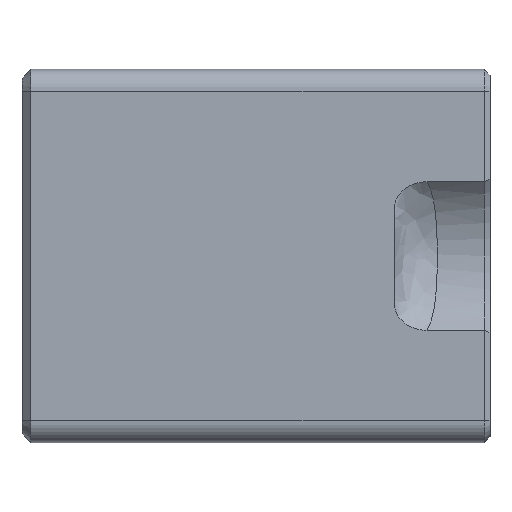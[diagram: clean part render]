
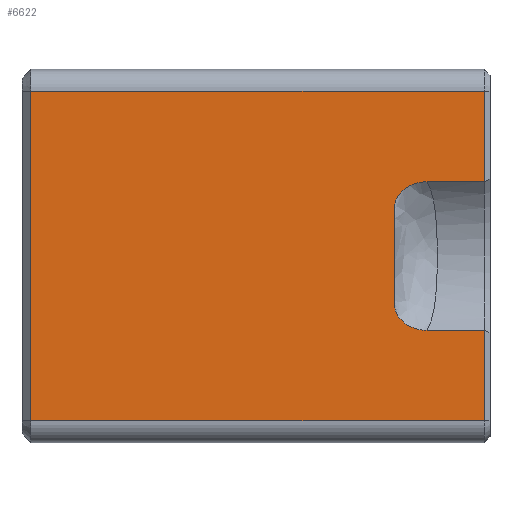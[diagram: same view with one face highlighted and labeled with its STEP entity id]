
A CAD part, front view. The second image highlights one B-rep face of the part: STEP entity #6622.
In plain terms, the highlighted planar face has unit normal (0, -1, 0).
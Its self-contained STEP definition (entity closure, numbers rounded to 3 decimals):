
#602=B_SPLINE_CURVE_WITH_KNOTS('',3,(#15782,#15783,#15784,#15785,#15786,
#15787,#15788,#15789,#15790,#15791,#15792,#15793,#15794,#15795,#15796,#15797,
#15798,#15799,#15800,#15801),.UNSPECIFIED.,.F.,.F.,(4,2,2,2,2,2,2,2,2,4),
(0.,0.,0.,0.002,0.007,
0.018,0.04,0.085,0.157,
0.234),.UNSPECIFIED.);
#603=B_SPLINE_CURVE_WITH_KNOTS('',3,(#15805,#15806,#15807,#15808,#15809,
#15810,#15811,#15812,#15813,#15814,#15815,#15816,#15817,#15818,#15819,#15820,
#15821,#15822,#15823,#15824),.UNSPECIFIED.,.F.,.F.,(4,2,2,2,2,2,2,2,2,4),
(0.,0.102,0.197,0.257,0.286,
0.3,0.306,0.31,0.31,
0.31),.UNSPECIFIED.);
#751=PLANE('',#7145);
#1197=FACE_OUTER_BOUND('',#1611,.T.);
#1611=EDGE_LOOP('',(#5960,#5961,#5962,#5963,#5964,#5965,#5966,#5967,#5968,
#5969));
#1972=LINE('',#15749,#2325);
#1981=LINE('',#15771,#2334);
#1982=LINE('',#15776,#2335);
#1983=LINE('',#15780,#2336);
#1984=LINE('',#15803,#2337);
#1985=LINE('',#15825,#2338);
#1986=LINE('',#15827,#2339);
#1987=LINE('',#15828,#2340);
#2325=VECTOR('',#8347,10.);
#2334=VECTOR('',#8380,10.);
#2335=VECTOR('',#8387,10.);
#2336=VECTOR('',#8392,10.);
#2337=VECTOR('',#8393,10.);
#2338=VECTOR('',#8394,10.);
#2339=VECTOR('',#8395,10.);
#2340=VECTOR('',#8396,10.);
#3175=VERTEX_POINT('',#15736);
#3176=VERTEX_POINT('',#15741);
#3177=VERTEX_POINT('',#15748);
#3178=VERTEX_POINT('',#15767);
#3179=VERTEX_POINT('',#15775);
#3180=VERTEX_POINT('',#15779);
#3181=VERTEX_POINT('',#15781);
#3182=VERTEX_POINT('',#15802);
#3183=VERTEX_POINT('',#15804);
#3184=VERTEX_POINT('',#15826);
#4108=EDGE_CURVE('',#3176,#3177,#1972,.T.);
#4121=EDGE_CURVE('',#3178,#3175,#1981,.T.);
#4123=EDGE_CURVE('',#3177,#3179,#1982,.T.);
#4125=EDGE_CURVE('',#3176,#3180,#1983,.T.);
#4126=EDGE_CURVE('',#3181,#3180,#602,.T.);
#4127=EDGE_CURVE('',#3181,#3182,#1984,.T.);
#4128=EDGE_CURVE('',#3182,#3183,#603,.F.);
#4129=EDGE_CURVE('',#3183,#3175,#1985,.T.);
#4130=EDGE_CURVE('',#3184,#3178,#1986,.T.);
#4131=EDGE_CURVE('',#3179,#3184,#1987,.T.);
#5960=ORIENTED_EDGE('',*,*,#4108,.F.);
#5961=ORIENTED_EDGE('',*,*,#4125,.T.);
#5962=ORIENTED_EDGE('',*,*,#4126,.F.);
#5963=ORIENTED_EDGE('',*,*,#4127,.T.);
#5964=ORIENTED_EDGE('',*,*,#4128,.T.);
#5965=ORIENTED_EDGE('',*,*,#4129,.T.);
#5966=ORIENTED_EDGE('',*,*,#4121,.F.);
#5967=ORIENTED_EDGE('',*,*,#4130,.F.);
#5968=ORIENTED_EDGE('',*,*,#4131,.F.);
#5969=ORIENTED_EDGE('',*,*,#4123,.F.);
#6622=ADVANCED_FACE('',(#1197),#751,.T.);
#7145=AXIS2_PLACEMENT_3D('',#15778,#8390,#8391);
#8347=DIRECTION('',(0.,0.,-1.));
#8380=DIRECTION('',(0.,0.,-1.));
#8387=DIRECTION('',(-1.,0.,0.));
#8390=DIRECTION('center_axis',(0.,-1.,0.));
#8391=DIRECTION('ref_axis',(0.,0.,1.));
#8392=DIRECTION('',(-1.,0.,0.));
#8393=DIRECTION('',(0.,0.,1.));
#8394=DIRECTION('',(1.,0.,0.));
#8395=DIRECTION('',(1.,0.,0.));
#8396=DIRECTION('',(0.,0.,1.));
#15736=CARTESIAN_POINT('',(-183.534,-11.455,5.083));
#15741=CARTESIAN_POINT('',(-183.534,-11.455,-5.083));
#15748=CARTESIAN_POINT('',(-183.534,-11.455,-11.264));
#15749=CARTESIAN_POINT('',(-183.534,-11.455,-6.128));
#15767=CARTESIAN_POINT('',(-183.534,-11.455,11.264));
#15771=CARTESIAN_POINT('',(-183.534,-11.455,-6.128));
#15775=CARTESIAN_POINT('',(-214.534,-11.455,-11.264));
#15776=CARTESIAN_POINT('',(-183.134,-11.455,-11.264));
#15778=CARTESIAN_POINT('Origin',(-183.134,-11.455,-12.256));
#15779=CARTESIAN_POINT('',(-187.44,-11.455,-5.083));
#15780=CARTESIAN_POINT('',(-183.134,-11.455,-5.083));
#15781=CARTESIAN_POINT('',(-189.634,-11.455,-3.546));
#15782=CARTESIAN_POINT('Ctrl Pts',(-189.634,-11.455,-3.546));
#15783=CARTESIAN_POINT('Ctrl Pts',(-189.634,-11.455,-3.546));
#15784=CARTESIAN_POINT('Ctrl Pts',(-189.634,-11.455,-3.547));
#15785=CARTESIAN_POINT('Ctrl Pts',(-189.634,-11.455,-3.548));
#15786=CARTESIAN_POINT('Ctrl Pts',(-189.634,-11.455,-3.549));
#15787=CARTESIAN_POINT('Ctrl Pts',(-189.634,-11.455,-3.558));
#15788=CARTESIAN_POINT('Ctrl Pts',(-189.633,-11.455,-3.566));
#15789=CARTESIAN_POINT('Ctrl Pts',(-189.63,-11.455,-3.592));
#15790=CARTESIAN_POINT('Ctrl Pts',(-189.627,-11.455,-3.61));
#15791=CARTESIAN_POINT('Ctrl Pts',(-189.616,-11.455,-3.667));
#15792=CARTESIAN_POINT('Ctrl Pts',(-189.605,-11.455,-3.707));
#15793=CARTESIAN_POINT('Ctrl Pts',(-189.566,-11.455,-3.826));
#15794=CARTESIAN_POINT('Ctrl Pts',(-189.531,-11.455,-3.905));
#15795=CARTESIAN_POINT('Ctrl Pts',(-189.407,-11.455,-4.136));
#15796=CARTESIAN_POINT('Ctrl Pts',(-189.297,-11.455,
-4.279));
#15797=CARTESIAN_POINT('Ctrl Pts',(-188.973,-11.455,
-4.603));
#15798=CARTESIAN_POINT('Ctrl Pts',(-188.724,-11.455,-4.771));
#15799=CARTESIAN_POINT('Ctrl Pts',(-188.119,-11.455,-5.02));
#15800=CARTESIAN_POINT('Ctrl Pts',(-187.781,-11.455,-5.083));
#15801=CARTESIAN_POINT('Ctrl Pts',(-187.44,-11.455,-5.083));
#15802=CARTESIAN_POINT('',(-189.634,-11.455,3.546));
#15803=CARTESIAN_POINT('',(-189.634,-11.455,-6.128));
#15804=CARTESIAN_POINT('',(-187.44,-11.455,5.083));
#15805=CARTESIAN_POINT('Ctrl Pts',(-187.44,-11.455,5.083));
#15806=CARTESIAN_POINT('Ctrl Pts',(-187.781,-11.455,5.083));
#15807=CARTESIAN_POINT('Ctrl Pts',(-188.119,-11.455,5.02));
#15808=CARTESIAN_POINT('Ctrl Pts',(-188.724,-11.455,4.771));
#15809=CARTESIAN_POINT('Ctrl Pts',(-188.973,-11.455,
4.603));
#15810=CARTESIAN_POINT('Ctrl Pts',(-189.297,-11.455,
4.279));
#15811=CARTESIAN_POINT('Ctrl Pts',(-189.407,-11.455,4.136));
#15812=CARTESIAN_POINT('Ctrl Pts',(-189.531,-11.455,3.905));
#15813=CARTESIAN_POINT('Ctrl Pts',(-189.566,-11.455,3.826));
#15814=CARTESIAN_POINT('Ctrl Pts',(-189.605,-11.455,3.707));
#15815=CARTESIAN_POINT('Ctrl Pts',(-189.616,-11.455,3.667));
#15816=CARTESIAN_POINT('Ctrl Pts',(-189.627,-11.455,3.61));
#15817=CARTESIAN_POINT('Ctrl Pts',(-189.63,-11.455,3.592));
#15818=CARTESIAN_POINT('Ctrl Pts',(-189.633,-11.455,3.565));
#15819=CARTESIAN_POINT('Ctrl Pts',(-189.634,-11.455,3.557));
#15820=CARTESIAN_POINT('Ctrl Pts',(-189.634,-11.455,3.549));
#15821=CARTESIAN_POINT('Ctrl Pts',(-189.634,-11.455,3.548));
#15822=CARTESIAN_POINT('Ctrl Pts',(-189.634,-11.455,3.547));
#15823=CARTESIAN_POINT('Ctrl Pts',(-189.634,-11.455,3.546));
#15824=CARTESIAN_POINT('Ctrl Pts',(-189.634,-11.455,3.546));
#15825=CARTESIAN_POINT('',(-183.134,-11.455,5.083));
#15826=CARTESIAN_POINT('',(-214.534,-11.455,11.264));
#15827=CARTESIAN_POINT('',(-183.134,-11.455,11.264));
#15828=CARTESIAN_POINT('',(-214.534,-11.455,-6.128));
